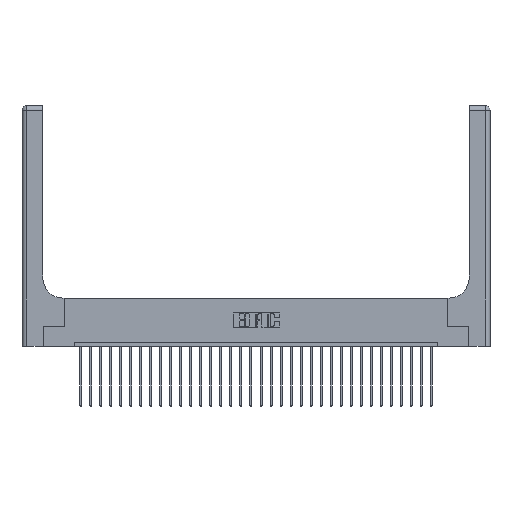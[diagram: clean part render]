
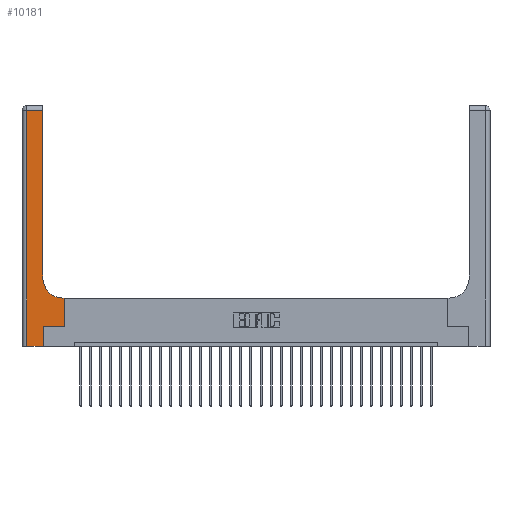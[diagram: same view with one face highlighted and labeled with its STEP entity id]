
A CAD part, top view. The second image highlights one B-rep face of the part: STEP entity #10181.
In plain terms, the highlighted planar face has unit normal (0, 0, 1).
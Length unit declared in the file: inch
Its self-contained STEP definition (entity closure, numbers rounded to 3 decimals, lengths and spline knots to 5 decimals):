
#217 = LINE ( 'NONE', #7054, #15985 ) ;
#371 = VECTOR ( 'NONE', #22090, 39.37008 ) ;
#379 = DIRECTION ( 'NONE',  ( 0., 1., 0. ) ) ;
#698 = DIRECTION ( 'NONE',  ( -1., 0., 0. ) ) ;
#882 = DIRECTION ( 'NONE',  ( 1., 0., 0. ) ) ;
#1139 = CARTESIAN_POINT ( 'NONE',  ( 0.26, 0.6, 0.37 ) ) ;
#2012 = ORIENTED_EDGE ( 'NONE', *, *, #19964, .T. ) ;
#3789 = CARTESIAN_POINT ( 'NONE',  ( 0.26, 2.94, 0.37 ) ) ;
#3989 = CARTESIAN_POINT ( 'NONE',  ( 0.06, 3., 0.37 ) ) ;
#4187 = ORIENTED_EDGE ( 'NONE', *, *, #18960, .T. ) ;
#4285 = LINE ( 'NONE', #3989, #8925 ) ;
#5104 = CARTESIAN_POINT ( 'NONE',  ( 0.265, 0., 0.37 ) ) ;
#5165 = AXIS2_PLACEMENT_3D ( 'NONE', #7361, #16271, #698 ) ;
#6617 = ORIENTED_EDGE ( 'NONE', *, *, #19231, .T. ) ;
#7054 = CARTESIAN_POINT ( 'NONE',  ( 0.265, 0.25, 0.37 ) ) ;
#7126 = VECTOR ( 'NONE', #379, 39.37008 ) ;
#7361 = CARTESIAN_POINT ( 'NONE',  ( 0., 3., 0.37 ) ) ;
#7495 = EDGE_CURVE ( 'NONE', #27721, #28350, #24737, .T. ) ;
#7565 = CARTESIAN_POINT ( 'NONE',  ( 0.528, 0.25, 0.37 ) ) ;
#7644 = EDGE_CURVE ( 'NONE', #13910, #14909, #17310, .T. ) ;
#8050 = ORIENTED_EDGE ( 'NONE', *, *, #11544, .T. ) ;
#8131 = CARTESIAN_POINT ( 'NONE',  ( 0., 2.94, 0.37 ) ) ;
#8925 = VECTOR ( 'NONE', #13305, 39.37008 ) ;
#9499 = VERTEX_POINT ( 'NONE', #16284 ) ;
#9840 = EDGE_LOOP ( 'NONE', ( #4187, #14842, #22984, #8050, #20380, #6617, #26709, #24569, #2012 ) ) ;
#10181 = ADVANCED_FACE ( 'NONE', ( #27344 ), #14239, .F. ) ;
#10694 = DIRECTION ( 'NONE',  ( -1., 0., 0. ) ) ;
#10942 = CARTESIAN_POINT ( 'NONE',  ( 0.26, 0.85, 0.37 ) ) ;
#11230 = CARTESIAN_POINT ( 'NONE',  ( 0.51, 0.6, 0.37 ) ) ;
#11544 = EDGE_CURVE ( 'NONE', #23796, #27721, #24971, .T. ) ;
#11836 = CARTESIAN_POINT ( 'NONE',  ( 0.528, 0.25, 0.37 ) ) ;
#11876 = DIRECTION ( 'NONE',  ( 1., 0., 0. ) ) ;
#11909 = LINE ( 'NONE', #1139, #21604 ) ;
#12001 = VECTOR ( 'NONE', #16037, 39.37008 ) ;
#12220 = AXIS2_PLACEMENT_3D ( 'NONE', #25637, #16330, #882 ) ;
#12555 = EDGE_CURVE ( 'NONE', #14909, #23796, #4285, .T. ) ;
#12658 = CARTESIAN_POINT ( 'NONE',  ( 0.265, 0., 0.37 ) ) ;
#13305 = DIRECTION ( 'NONE',  ( 0., -1., 0. ) ) ;
#13910 = VERTEX_POINT ( 'NONE', #3789 ) ;
#14007 = VECTOR ( 'NONE', #11876, 39.37008 ) ;
#14239 = PLANE ( 'NONE',  #5165 ) ;
#14842 = ORIENTED_EDGE ( 'NONE', *, *, #7644, .T. ) ;
#14909 = VERTEX_POINT ( 'NONE', #16544 ) ;
#15521 = DIRECTION ( 'NONE',  ( 0., 1., 0. ) ) ;
#15968 = DIRECTION ( 'NONE',  ( 1., 0., 0. ) ) ;
#15985 = VECTOR ( 'NONE', #15968, 39.37008 ) ;
#16037 = DIRECTION ( 'NONE',  ( 0., 1., 0. ) ) ;
#16271 = DIRECTION ( 'NONE',  ( 0., 0., -1. ) ) ;
#16284 = CARTESIAN_POINT ( 'NONE',  ( 0.528, 0.6, 0.37 ) ) ;
#16330 = DIRECTION ( 'NONE',  ( 0., 0., -1. ) ) ;
#16380 = CARTESIAN_POINT ( 'NONE',  ( 0.265, 0.25, 0.37 ) ) ;
#16544 = CARTESIAN_POINT ( 'NONE',  ( 0.06, 2.94, 0.37 ) ) ;
#17310 = LINE ( 'NONE', #8131, #371 ) ;
#18960 = EDGE_CURVE ( 'NONE', #26951, #13910, #23093, .T. ) ;
#19231 = EDGE_CURVE ( 'NONE', #28350, #26395, #217, .T. ) ;
#19964 = EDGE_CURVE ( 'NONE', #23461, #26951, #23358, .T. ) ;
#20380 = ORIENTED_EDGE ( 'NONE', *, *, #7495, .T. ) ;
#20640 = VECTOR ( 'NONE', #15521, 39.37008 ) ;
#21604 = VECTOR ( 'NONE', #10694, 39.37008 ) ;
#22090 = DIRECTION ( 'NONE',  ( -1., 0., 0. ) ) ;
#22984 = ORIENTED_EDGE ( 'NONE', *, *, #12555, .T. ) ;
#23093 = LINE ( 'NONE', #27201, #7126 ) ;
#23358 = CIRCLE ( 'NONE', #12220, 0.25 ) ;
#23461 = VERTEX_POINT ( 'NONE', #11230 ) ;
#23516 = CARTESIAN_POINT ( 'NONE',  ( 0.06, 0., 0.37 ) ) ;
#23796 = VERTEX_POINT ( 'NONE', #23516 ) ;
#24515 = LINE ( 'NONE', #7565, #20640 ) ;
#24569 = ORIENTED_EDGE ( 'NONE', *, *, #26274, .T. ) ;
#24737 = LINE ( 'NONE', #5104, #12001 ) ;
#24971 = LINE ( 'NONE', #27313, #14007 ) ;
#25637 = CARTESIAN_POINT ( 'NONE',  ( 0.51, 0.85, 0.37 ) ) ;
#26274 = EDGE_CURVE ( 'NONE', #9499, #23461, #11909, .T. ) ;
#26395 = VERTEX_POINT ( 'NONE', #11836 ) ;
#26709 = ORIENTED_EDGE ( 'NONE', *, *, #27654, .T. ) ;
#26951 = VERTEX_POINT ( 'NONE', #10942 ) ;
#27201 = CARTESIAN_POINT ( 'NONE',  ( 0.26, 3., 0.37 ) ) ;
#27313 = CARTESIAN_POINT ( 'NONE',  ( 0., 0., 0.37 ) ) ;
#27344 = FACE_OUTER_BOUND ( 'NONE', #9840, .T. ) ;
#27654 = EDGE_CURVE ( 'NONE', #26395, #9499, #24515, .T. ) ;
#27721 = VERTEX_POINT ( 'NONE', #12658 ) ;
#28350 = VERTEX_POINT ( 'NONE', #16380 ) ;
